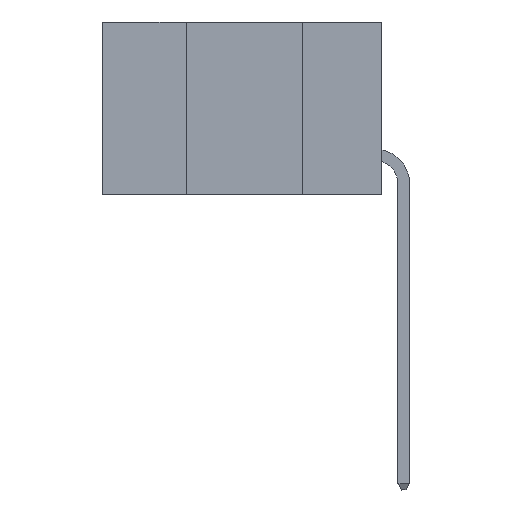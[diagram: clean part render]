
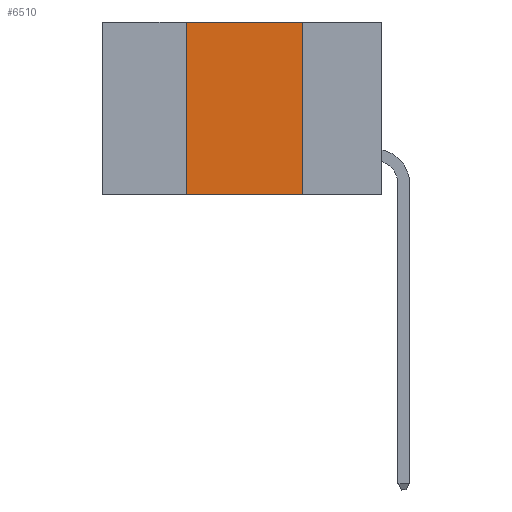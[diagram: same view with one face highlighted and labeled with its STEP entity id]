
A CAD part, left-side view. The second image highlights one B-rep face of the part: STEP entity #6510.
In plain terms, the highlighted planar face has unit normal (-1, 0, 0).
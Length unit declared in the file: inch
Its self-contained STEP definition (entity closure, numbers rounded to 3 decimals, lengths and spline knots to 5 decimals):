
#70 = EDGE_CURVE ( 'NONE', #10664, #24214, #24978, .T. ) ;
#220 = VECTOR ( 'NONE', #10151, 39.37008 ) ;
#486 = CARTESIAN_POINT ( 'NONE',  ( 0., 0.6, 0. ) ) ;
#1136 = LINE ( 'NONE', #4506, #6517 ) ;
#2444 = ORIENTED_EDGE ( 'NONE', *, *, #13718, .F. ) ;
#4506 = CARTESIAN_POINT ( 'NONE',  ( 0., 0.42, 0. ) ) ;
#5412 = ORIENTED_EDGE ( 'NONE', *, *, #8872, .F. ) ;
#6510 = ADVANCED_FACE ( 'NONE', ( #19351 ), #17617, .F. ) ;
#6517 = VECTOR ( 'NONE', #17931, 39.37008 ) ;
#8232 = AXIS2_PLACEMENT_3D ( 'NONE', #23437, #14185, #12841 ) ;
#8872 = EDGE_CURVE ( 'NONE', #24214, #12811, #12560, .T. ) ;
#10151 = DIRECTION ( 'NONE',  ( 0., -1., 0. ) ) ;
#10664 = VERTEX_POINT ( 'NONE', #22130 ) ;
#11290 = CARTESIAN_POINT ( 'NONE',  ( 0., 0.17, 0. ) ) ;
#12039 = CARTESIAN_POINT ( 'NONE',  ( 0., 0.6, -0.37 ) ) ;
#12560 = LINE ( 'NONE', #24934, #14349 ) ;
#12811 = VERTEX_POINT ( 'NONE', #20708 ) ;
#12841 = DIRECTION ( 'NONE',  ( 0., 0., -1. ) ) ;
#13718 = EDGE_CURVE ( 'NONE', #17884, #10664, #1136, .T. ) ;
#14185 = DIRECTION ( 'NONE',  ( 1., 0., 0. ) ) ;
#14349 = VECTOR ( 'NONE', #24697, 39.37008 ) ;
#15929 = CARTESIAN_POINT ( 'NONE',  ( 0., 0.42, -0.37 ) ) ;
#17184 = LINE ( 'NONE', #12039, #21398 ) ;
#17617 = PLANE ( 'NONE',  #8232 ) ;
#17884 = VERTEX_POINT ( 'NONE', #15929 ) ;
#17931 = DIRECTION ( 'NONE',  ( 0., 0., 1. ) ) ;
#18869 = ORIENTED_EDGE ( 'NONE', *, *, #24810, .T. ) ;
#19351 = FACE_OUTER_BOUND ( 'NONE', #23187, .T. ) ;
#19876 = DIRECTION ( 'NONE',  ( 0., -1., 0. ) ) ;
#20708 = CARTESIAN_POINT ( 'NONE',  ( 0., 0.17, -0.37 ) ) ;
#21398 = VECTOR ( 'NONE', #19876, 39.37008 ) ;
#22130 = CARTESIAN_POINT ( 'NONE',  ( 0., 0.42, 0. ) ) ;
#23187 = EDGE_LOOP ( 'NONE', ( #5412, #24962, #2444, #18869 ) ) ;
#23437 = CARTESIAN_POINT ( 'NONE',  ( 0., 0.6, 0. ) ) ;
#24214 = VERTEX_POINT ( 'NONE', #11290 ) ;
#24697 = DIRECTION ( 'NONE',  ( 0., 0., -1. ) ) ;
#24810 = EDGE_CURVE ( 'NONE', #17884, #12811, #17184, .T. ) ;
#24934 = CARTESIAN_POINT ( 'NONE',  ( 0., 0.17, 0. ) ) ;
#24962 = ORIENTED_EDGE ( 'NONE', *, *, #70, .F. ) ;
#24978 = LINE ( 'NONE', #486, #220 ) ;
